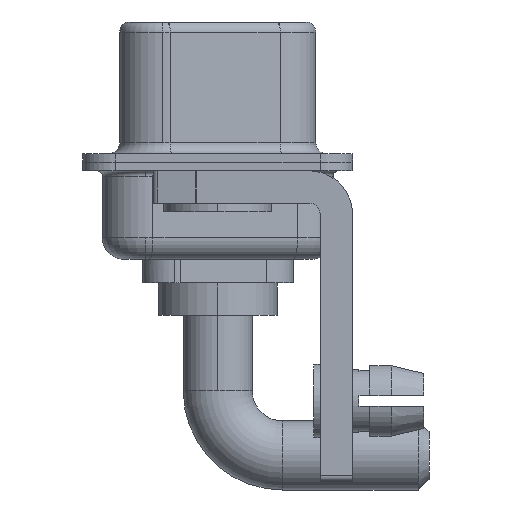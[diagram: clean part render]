
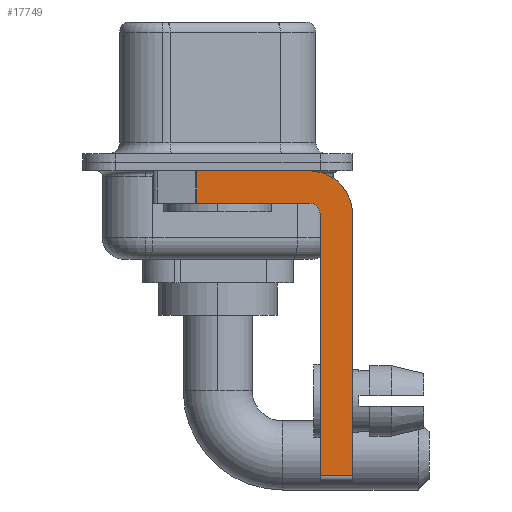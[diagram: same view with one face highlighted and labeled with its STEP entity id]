
A CAD part, left-side view. The second image highlights one B-rep face of the part: STEP entity #17749.
In plain terms, the highlighted planar face has unit normal (-1, 0, 0).
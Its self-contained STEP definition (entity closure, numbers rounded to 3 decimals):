
#92 = DIRECTION ( 'NONE',  ( 0., 0., -1. ) ) ;
#357 = CARTESIAN_POINT ( 'NONE',  ( -2.9, -4.75, -14.55 ) ) ;
#703 = CARTESIAN_POINT ( 'NONE',  ( -2.9, -4.25, -0.4 ) ) ;
#859 = LINE ( 'NONE', #11124, #4456 ) ;
#1101 = VECTOR ( 'NONE', #10453, 1000. ) ;
#1273 = ORIENTED_EDGE ( 'NONE', *, *, #17253, .T. ) ;
#1365 = CARTESIAN_POINT ( 'NONE',  ( -2.9, -4.25, -2.4 ) ) ;
#1410 = CARTESIAN_POINT ( 'NONE',  ( -2.9, -4.75, -2.4 ) ) ;
#1416 = VERTEX_POINT ( 'NONE', #15014 ) ;
#2219 = DIRECTION ( 'NONE',  ( 0., 1., 0. ) ) ;
#2568 = PLANE ( 'NONE',  #8400 ) ;
#2725 = DIRECTION ( 'NONE',  ( 0., 0., -1. ) ) ;
#2797 = VECTOR ( 'NONE', #2725, 1000. ) ;
#3751 = VERTEX_POINT ( 'NONE', #1410 ) ;
#3968 = VERTEX_POINT ( 'NONE', #9681 ) ;
#4252 = LINE ( 'NONE', #8531, #16191 ) ;
#4456 = VECTOR ( 'NONE', #10943, 1000. ) ;
#4521 = EDGE_CURVE ( 'NONE', #3968, #13803, #9196, .T. ) ;
#4714 = LINE ( 'NONE', #6402, #16616 ) ;
#5526 = CARTESIAN_POINT ( 'NONE',  ( -2.9, 3., -0.4 ) ) ;
#5830 = DIRECTION ( 'NONE',  ( 0., -1., 0. ) ) ;
#6272 = DIRECTION ( 'NONE',  ( -1., 0., 0. ) ) ;
#6373 = CARTESIAN_POINT ( 'NONE',  ( -2.9, -4.25, -2.4 ) ) ;
#6402 = CARTESIAN_POINT ( 'NONE',  ( -2.9, -4.25, -1.9 ) ) ;
#6485 = VERTEX_POINT ( 'NONE', #14446 ) ;
#6616 = AXIS2_PLACEMENT_3D ( 'NONE', #9975, #12884, #92 ) ;
#6741 = DIRECTION ( 'NONE',  ( 0., -1., 0. ) ) ;
#7438 = ORIENTED_EDGE ( 'NONE', *, *, #14774, .F. ) ;
#7456 = EDGE_LOOP ( 'NONE', ( #9488, #12035, #9710, #9271, #7438, #1273, #15980, #10267 ) ) ;
#7644 = EDGE_CURVE ( 'NONE', #3968, #1416, #9806, .T. ) ;
#7972 = VERTEX_POINT ( 'NONE', #11101 ) ;
#8400 = AXIS2_PLACEMENT_3D ( 'NONE', #1365, #17053, #15658 ) ;
#8531 = CARTESIAN_POINT ( 'NONE',  ( -2.9, -4.25, -14.55 ) ) ;
#8569 = CARTESIAN_POINT ( 'NONE',  ( -2.9, 0.978, -1.9 ) ) ;
#9196 = LINE ( 'NONE', #5526, #11341 ) ;
#9271 = ORIENTED_EDGE ( 'NONE', *, *, #16046, .F. ) ;
#9488 = ORIENTED_EDGE ( 'NONE', *, *, #4521, .F. ) ;
#9681 = CARTESIAN_POINT ( 'NONE',  ( -2.9, 0.978, -0.4 ) ) ;
#9710 = ORIENTED_EDGE ( 'NONE', *, *, #12172, .F. ) ;
#9806 = LINE ( 'NONE', #8569, #2797 ) ;
#9975 = CARTESIAN_POINT ( 'NONE',  ( -2.9, -4.25, -2.4 ) ) ;
#10267 = ORIENTED_EDGE ( 'NONE', *, *, #18370, .F. ) ;
#10385 = DIRECTION ( 'NONE',  ( 0., 0., 1. ) ) ;
#10453 = DIRECTION ( 'NONE',  ( 0., 0., -1. ) ) ;
#10943 = DIRECTION ( 'NONE',  ( 0., 0., 1. ) ) ;
#11101 = CARTESIAN_POINT ( 'NONE',  ( -2.9, -4.25, -1.9 ) ) ;
#11124 = CARTESIAN_POINT ( 'NONE',  ( -2.9, -4.75, -14.8 ) ) ;
#11341 = VECTOR ( 'NONE', #6741, 1000. ) ;
#11867 = CARTESIAN_POINT ( 'NONE',  ( -2.9, -6.25, -2.4 ) ) ;
#12035 = ORIENTED_EDGE ( 'NONE', *, *, #7644, .T. ) ;
#12172 = EDGE_CURVE ( 'NONE', #7972, #1416, #4714, .T. ) ;
#12450 = CARTESIAN_POINT ( 'NONE',  ( -2.9, -6.25, -14.55 ) ) ;
#12884 = DIRECTION ( 'NONE',  ( 1., 0., 0. ) ) ;
#13169 = AXIS2_PLACEMENT_3D ( 'NONE', #6373, #6272, #10385 ) ;
#13654 = LINE ( 'NONE', #11867, #1101 ) ;
#13803 = VERTEX_POINT ( 'NONE', #703 ) ;
#14091 = CIRCLE ( 'NONE', #6616, 2. ) ;
#14182 = EDGE_CURVE ( 'NONE', #6485, #16194, #13654, .T. ) ;
#14446 = CARTESIAN_POINT ( 'NONE',  ( -2.9, -6.25, -2.4 ) ) ;
#14774 = EDGE_CURVE ( 'NONE', #17012, #3751, #859, .T. ) ;
#15014 = CARTESIAN_POINT ( 'NONE',  ( -2.9, 0.978, -1.9 ) ) ;
#15564 = CIRCLE ( 'NONE', #13169, 0.5 ) ;
#15658 = DIRECTION ( 'NONE',  ( 0., 0., -1. ) ) ;
#15980 = ORIENTED_EDGE ( 'NONE', *, *, #14182, .F. ) ;
#16046 = EDGE_CURVE ( 'NONE', #3751, #7972, #15564, .T. ) ;
#16191 = VECTOR ( 'NONE', #5830, 1000. ) ;
#16194 = VERTEX_POINT ( 'NONE', #12450 ) ;
#16616 = VECTOR ( 'NONE', #2219, 1000. ) ;
#17012 = VERTEX_POINT ( 'NONE', #357 ) ;
#17053 = DIRECTION ( 'NONE',  ( 1., 0., 0. ) ) ;
#17253 = EDGE_CURVE ( 'NONE', #17012, #16194, #4252, .T. ) ;
#17749 = ADVANCED_FACE ( 'NONE', ( #18464 ), #2568, .F. ) ;
#18370 = EDGE_CURVE ( 'NONE', #13803, #6485, #14091, .T. ) ;
#18464 = FACE_OUTER_BOUND ( 'NONE', #7456, .T. ) ;
